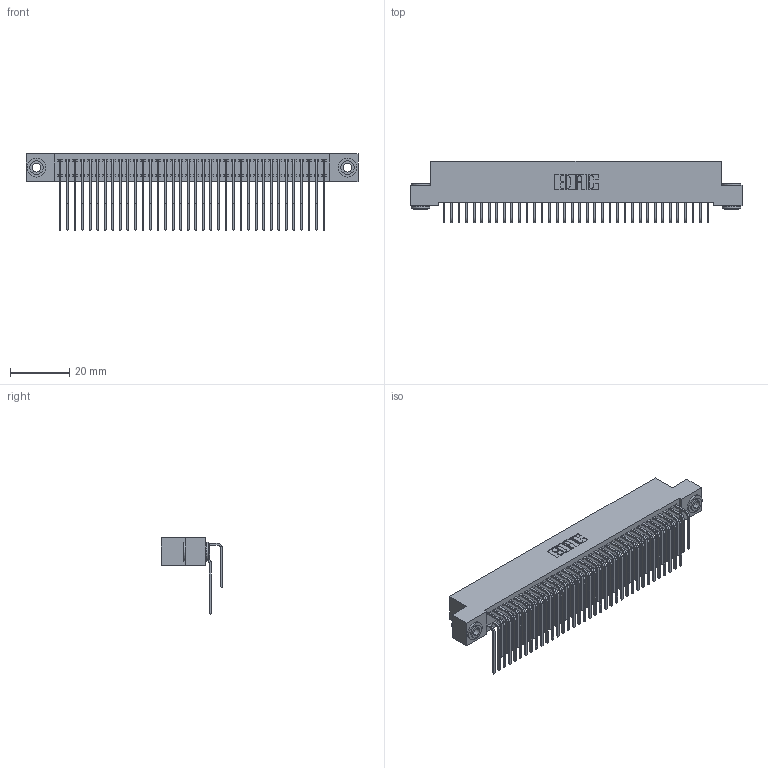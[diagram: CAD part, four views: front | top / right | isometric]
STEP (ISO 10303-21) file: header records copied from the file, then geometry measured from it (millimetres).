
FILE_DESCRIPTION (( 'STEP AP203' ), '1' );
FILE_NAME ('392-072-559-203.STEP', '2018-08-18T00:25:27', ( '' ), ( '' ), 'SwSTEP 2.0', 'SolidWorks 2016', '' );
FILE_SCHEMA (( 'CONFIG_CONTROL_DESIGN' ));
Length unit declared in the file: inch
Products named in the file (5): 345-292-001_558 559 Tail - 1; 345-292-001_559 Tail - 2; 342-250-002_345-250-002-102; 392-072-559-203; 342 Part_.156 TH
Assembly tree (75 placements, depth 2):
  392-072-559-203
    342 Part_.156 TH
    345-292-001_558 559 Tail - 1  x36
    345-292-001_559 Tail - 2  x36
    342-250-002_345-250-002-102  x2
Bounding box: 111.76 x 20.64 x 25.78 mm (x, y, z)
Volume: 10451.4 mm3; surface area: 18957.4 mm2
Topology: 75 solids, 75 shells, 4036 faces, 11967 edges, 7878 vertices
Faces by surface type: plane 2812, cylinder 1216, cone 8
Entity records: 26238 total; most frequent: CARTESIAN_POINT 4380, ORIENTED_EDGE 4258, DIRECTION 3767, EDGE_CURVE 2129, VECTOR 1937, LINE 1937, VERTEX_POINT 1414, AXIS2_PLACEMENT_3D 915
